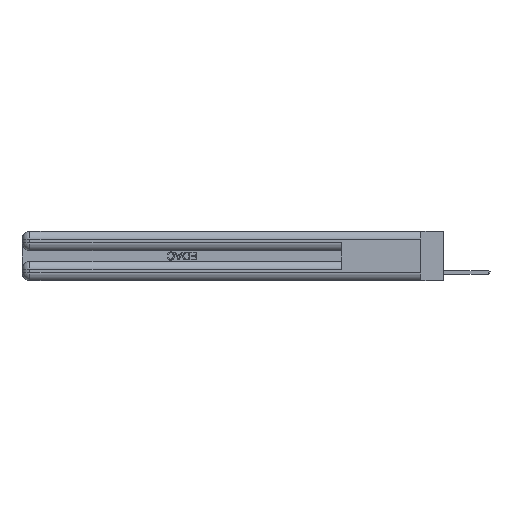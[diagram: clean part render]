
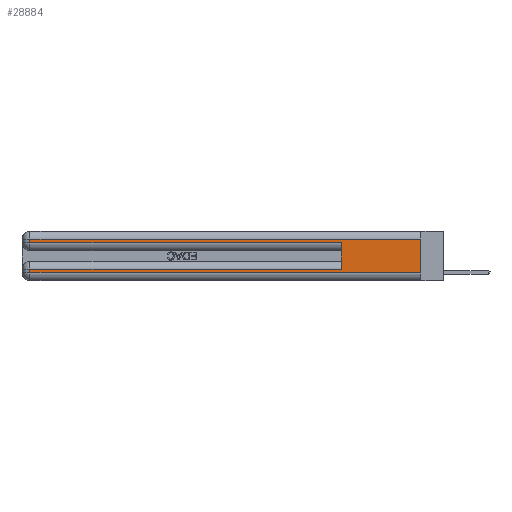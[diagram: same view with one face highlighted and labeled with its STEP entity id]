
A CAD part, left-side view. The second image highlights one B-rep face of the part: STEP entity #28884.
In plain terms, the highlighted planar face has unit normal (-1, 0, 0).
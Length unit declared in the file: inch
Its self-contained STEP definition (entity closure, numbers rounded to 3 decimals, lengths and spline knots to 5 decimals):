
#262 = CARTESIAN_POINT ( 'NONE',  ( 0., 0.6, 0.085 ) ) ;
#800 = EDGE_CURVE ( 'NONE', #7658, #23856, #27293, .T. ) ;
#849 = EDGE_CURVE ( 'NONE', #33775, #11992, #34897, .T. ) ;
#906 = CARTESIAN_POINT ( 'NONE',  ( 0., 0., 0.31 ) ) ;
#963 = DIRECTION ( 'NONE',  ( 0., -1., 0. ) ) ;
#986 = EDGE_LOOP ( 'NONE', ( #25442, #14765, #7184, #9510, #31363, #32160, #34152, #35057 ) ) ;
#1505 = VERTEX_POINT ( 'NONE', #34623 ) ;
#2587 = LINE ( 'NONE', #23175, #18911 ) ;
#3040 = DIRECTION ( 'NONE',  ( 1., 0., 0. ) ) ;
#3871 = EDGE_CURVE ( 'NONE', #23856, #1505, #26375, .T. ) ;
#4865 = VECTOR ( 'NONE', #24430, 39.37008 ) ;
#6163 = CARTESIAN_POINT ( 'NONE',  ( 0., 2.94, 0.31 ) ) ;
#7184 = ORIENTED_EDGE ( 'NONE', *, *, #3871, .T. ) ;
#7658 = VERTEX_POINT ( 'NONE', #14116 ) ;
#7675 = VECTOR ( 'NONE', #26982, 39.37008 ) ;
#8469 = AXIS2_PLACEMENT_3D ( 'NONE', #27039, #3040, #11181 ) ;
#9043 = VECTOR ( 'NONE', #25243, 39.37008 ) ;
#9296 = VECTOR ( 'NONE', #10992, 39.37008 ) ;
#9510 = ORIENTED_EDGE ( 'NONE', *, *, #15282, .T. ) ;
#10618 = LINE ( 'NONE', #22834, #15272 ) ;
#10992 = DIRECTION ( 'NONE',  ( 0., 0., -1. ) ) ;
#11181 = DIRECTION ( 'NONE',  ( 0., 0., -1. ) ) ;
#11885 = VECTOR ( 'NONE', #14786, 39.37008 ) ;
#11992 = VERTEX_POINT ( 'NONE', #25658 ) ;
#12786 = VERTEX_POINT ( 'NONE', #22689 ) ;
#13655 = CARTESIAN_POINT ( 'NONE',  ( 0., 0.6, 0.145 ) ) ;
#14116 = CARTESIAN_POINT ( 'NONE',  ( 0., 0., 0.31 ) ) ;
#14765 = ORIENTED_EDGE ( 'NONE', *, *, #800, .T. ) ;
#14786 = DIRECTION ( 'NONE',  ( 0., 0., -1. ) ) ;
#15272 = VECTOR ( 'NONE', #22378, 39.37008 ) ;
#15282 = EDGE_CURVE ( 'NONE', #1505, #18032, #10618, .T. ) ;
#17358 = VERTEX_POINT ( 'NONE', #262 ) ;
#17568 = EDGE_CURVE ( 'NONE', #17358, #18032, #34692, .T. ) ;
#18032 = VERTEX_POINT ( 'NONE', #34711 ) ;
#18911 = VECTOR ( 'NONE', #963, 39.37008 ) ;
#19797 = CARTESIAN_POINT ( 'NONE',  ( 0., 0., 0.085 ) ) ;
#21967 = FACE_OUTER_BOUND ( 'NONE', #986, .T. ) ;
#22053 = PLANE ( 'NONE',  #8469 ) ;
#22378 = DIRECTION ( 'NONE',  ( 0., -1., 0. ) ) ;
#22689 = CARTESIAN_POINT ( 'NONE',  ( 0., 0., 0.06 ) ) ;
#22770 = DIRECTION ( 'NONE',  ( 0., 1., 0. ) ) ;
#22834 = CARTESIAN_POINT ( 'NONE',  ( 0., 0., 0.285 ) ) ;
#23175 = CARTESIAN_POINT ( 'NONE',  ( 0., 0., 0.06 ) ) ;
#23856 = VERTEX_POINT ( 'NONE', #6163 ) ;
#24430 = DIRECTION ( 'NONE',  ( 0., 0., 1. ) ) ;
#25243 = DIRECTION ( 'NONE',  ( 0., 1., 0. ) ) ;
#25442 = ORIENTED_EDGE ( 'NONE', *, *, #33271, .F. ) ;
#25658 = CARTESIAN_POINT ( 'NONE',  ( 0., 2.94, 0.06 ) ) ;
#26001 = VECTOR ( 'NONE', #22770, 39.37008 ) ;
#26375 = LINE ( 'NONE', #28347, #11885 ) ;
#26982 = DIRECTION ( 'NONE',  ( 0., 0., -1. ) ) ;
#27039 = CARTESIAN_POINT ( 'NONE',  ( 0., 0., 0.37 ) ) ;
#27293 = LINE ( 'NONE', #906, #26001 ) ;
#28184 = LINE ( 'NONE', #19797, #9043 ) ;
#28347 = CARTESIAN_POINT ( 'NONE',  ( 0., 2.94, 0.37 ) ) ;
#28884 = ADVANCED_FACE ( 'NONE', ( #21967 ), #22053, .F. ) ;
#29832 = CARTESIAN_POINT ( 'NONE',  ( 0., 2.94, 0.37 ) ) ;
#31033 = LINE ( 'NONE', #32413, #9296 ) ;
#31363 = ORIENTED_EDGE ( 'NONE', *, *, #17568, .F. ) ;
#32160 = ORIENTED_EDGE ( 'NONE', *, *, #35087, .T. ) ;
#32413 = CARTESIAN_POINT ( 'NONE',  ( 0., 0., 0.37 ) ) ;
#32761 = CARTESIAN_POINT ( 'NONE',  ( 0., 2.94, 0.085 ) ) ;
#33271 = EDGE_CURVE ( 'NONE', #7658, #12786, #31033, .T. ) ;
#33775 = VERTEX_POINT ( 'NONE', #32761 ) ;
#34152 = ORIENTED_EDGE ( 'NONE', *, *, #849, .T. ) ;
#34623 = CARTESIAN_POINT ( 'NONE',  ( 0., 2.94, 0.285 ) ) ;
#34692 = LINE ( 'NONE', #13655, #4865 ) ;
#34711 = CARTESIAN_POINT ( 'NONE',  ( 0., 0.6, 0.285 ) ) ;
#34897 = LINE ( 'NONE', #29832, #7675 ) ;
#35057 = ORIENTED_EDGE ( 'NONE', *, *, #35221, .T. ) ;
#35087 = EDGE_CURVE ( 'NONE', #17358, #33775, #28184, .T. ) ;
#35221 = EDGE_CURVE ( 'NONE', #11992, #12786, #2587, .T. ) ;
